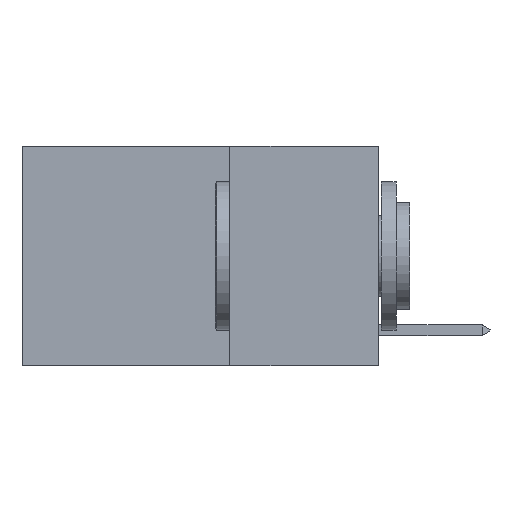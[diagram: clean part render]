
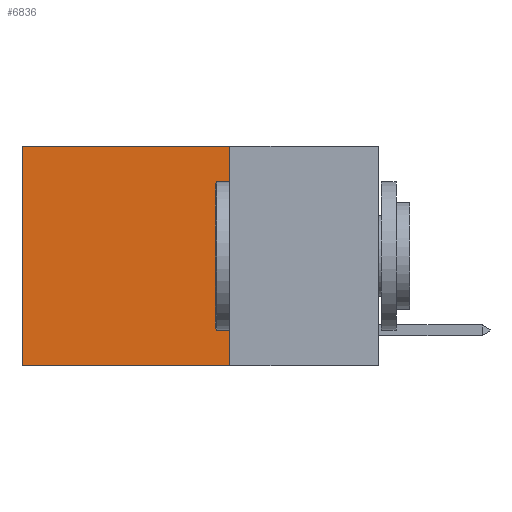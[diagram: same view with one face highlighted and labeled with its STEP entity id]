
A CAD part, left-side view. The second image highlights one B-rep face of the part: STEP entity #6836.
In plain terms, the highlighted planar face has unit normal (-1, 0, 0).
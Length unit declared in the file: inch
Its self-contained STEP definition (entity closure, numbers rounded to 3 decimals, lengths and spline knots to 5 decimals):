
#382 = DIRECTION ( 'NONE',  ( 0., 1., 0. ) ) ;
#1277 = DIRECTION ( 'NONE',  ( 0., 0., -1. ) ) ;
#1455 = LINE ( 'NONE', #22892, #19731 ) ;
#1714 = CARTESIAN_POINT ( 'NONE',  ( 0.2625, 0.6, -0.37 ) ) ;
#3128 = VECTOR ( 'NONE', #382, 39.37008 ) ;
#3270 = VECTOR ( 'NONE', #21455, 39.37008 ) ;
#3706 = CARTESIAN_POINT ( 'NONE',  ( 0.2625, 0.25, -0.37 ) ) ;
#4089 = VERTEX_POINT ( 'NONE', #1714 ) ;
#4168 = EDGE_CURVE ( 'NONE', #17766, #4089, #17370, .T. ) ;
#4363 = ORIENTED_EDGE ( 'NONE', *, *, #4168, .F. ) ;
#5724 = EDGE_LOOP ( 'NONE', ( #14575, #4363, #14298, #18269 ) ) ;
#6289 = VECTOR ( 'NONE', #17167, 39.37008 ) ;
#6438 = VERTEX_POINT ( 'NONE', #15746 ) ;
#6836 = ADVANCED_FACE ( 'NONE', ( #21745 ), #20715, .F. ) ;
#7406 = CARTESIAN_POINT ( 'NONE',  ( 0.2625, 0.6, 0. ) ) ;
#9806 = CARTESIAN_POINT ( 'NONE',  ( 0.2625, 0.25, -0.37 ) ) ;
#10122 = CARTESIAN_POINT ( 'NONE',  ( 0.2625, 0.25, 0. ) ) ;
#11895 = DIRECTION ( 'NONE',  ( 1., 0., 0. ) ) ;
#12442 = EDGE_CURVE ( 'NONE', #14902, #4089, #20443, .T. ) ;
#14298 = ORIENTED_EDGE ( 'NONE', *, *, #22352, .F. ) ;
#14575 = ORIENTED_EDGE ( 'NONE', *, *, #12442, .T. ) ;
#14902 = VERTEX_POINT ( 'NONE', #7406 ) ;
#15376 = CARTESIAN_POINT ( 'NONE',  ( 0.2625, 0.6, 0. ) ) ;
#15746 = CARTESIAN_POINT ( 'NONE',  ( 0.2625, 0.25, 0. ) ) ;
#17167 = DIRECTION ( 'NONE',  ( 0., 0., -1. ) ) ;
#17235 = LINE ( 'NONE', #21624, #3128 ) ;
#17258 = AXIS2_PLACEMENT_3D ( 'NONE', #10122, #11895, #1277 ) ;
#17370 = LINE ( 'NONE', #3706, #3270 ) ;
#17766 = VERTEX_POINT ( 'NONE', #9806 ) ;
#18269 = ORIENTED_EDGE ( 'NONE', *, *, #21285, .T. ) ;
#19332 = DIRECTION ( 'NONE',  ( 0., 0., -1. ) ) ;
#19731 = VECTOR ( 'NONE', #19332, 39.37008 ) ;
#20443 = LINE ( 'NONE', #15376, #6289 ) ;
#20715 = PLANE ( 'NONE',  #17258 ) ;
#21285 = EDGE_CURVE ( 'NONE', #6438, #14902, #17235, .T. ) ;
#21455 = DIRECTION ( 'NONE',  ( 0., 1., 0. ) ) ;
#21624 = CARTESIAN_POINT ( 'NONE',  ( 0.2625, 0.25, 0. ) ) ;
#21745 = FACE_OUTER_BOUND ( 'NONE', #5724, .T. ) ;
#22352 = EDGE_CURVE ( 'NONE', #6438, #17766, #1455, .T. ) ;
#22892 = CARTESIAN_POINT ( 'NONE',  ( 0.2625, 0.25, 0. ) ) ;
